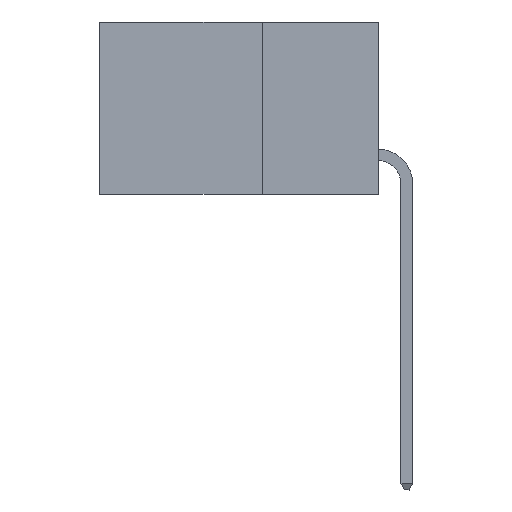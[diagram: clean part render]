
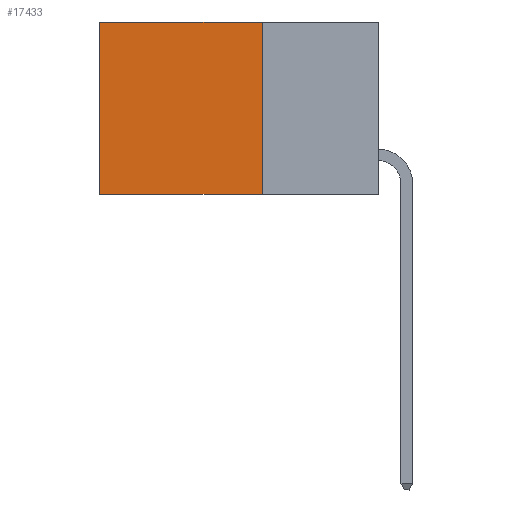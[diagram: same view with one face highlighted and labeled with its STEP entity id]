
A CAD part, left-side view. The second image highlights one B-rep face of the part: STEP entity #17433.
In plain terms, the highlighted planar face has unit normal (-1, 0, 0).
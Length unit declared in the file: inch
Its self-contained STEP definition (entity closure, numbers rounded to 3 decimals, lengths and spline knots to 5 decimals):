
#5151 = VECTOR ( 'NONE', #5388, 39.37008 ) ;
#5304 = CARTESIAN_POINT ( 'NONE',  ( 0.298, 0.25, 0. ) ) ;
#5388 = DIRECTION ( 'NONE',  ( 0., 1., 0. ) ) ;
#5449 = VECTOR ( 'NONE', #15391, 39.37008 ) ;
#6248 = CARTESIAN_POINT ( 'NONE',  ( 0.298, 0.6, 0. ) ) ;
#6338 = VERTEX_POINT ( 'NONE', #20935 ) ;
#7068 = ORIENTED_EDGE ( 'NONE', *, *, #19217, .F. ) ;
#7825 = ORIENTED_EDGE ( 'NONE', *, *, #17321, .T. ) ;
#8669 = EDGE_CURVE ( 'NONE', #17113, #14033, #10089, .T. ) ;
#9116 = VECTOR ( 'NONE', #25339, 39.37008 ) ;
#9495 = ORIENTED_EDGE ( 'NONE', *, *, #8669, .T. ) ;
#9577 = CARTESIAN_POINT ( 'NONE',  ( 0.298, 0.25, 0. ) ) ;
#10061 = EDGE_CURVE ( 'NONE', #6338, #14033, #15843, .T. ) ;
#10089 = LINE ( 'NONE', #6248, #9116 ) ;
#11891 = CARTESIAN_POINT ( 'NONE',  ( 0.298, 0.25, 0. ) ) ;
#12530 = CARTESIAN_POINT ( 'NONE',  ( 0.298, 0.6, 0. ) ) ;
#12676 = ORIENTED_EDGE ( 'NONE', *, *, #10061, .F. ) ;
#13396 = EDGE_LOOP ( 'NONE', ( #9495, #12676, #7068, #7825 ) ) ;
#13481 = CARTESIAN_POINT ( 'NONE',  ( 0.298, 0.25, -0.37 ) ) ;
#14033 = VERTEX_POINT ( 'NONE', #27015 ) ;
#15391 = DIRECTION ( 'NONE',  ( 0., 1., 0. ) ) ;
#15843 = LINE ( 'NONE', #13481, #5449 ) ;
#17113 = VERTEX_POINT ( 'NONE', #12530 ) ;
#17321 = EDGE_CURVE ( 'NONE', #18151, #17113, #27006, .T. ) ;
#17433 = ADVANCED_FACE ( 'NONE', ( #26339 ), #23922, .F. ) ;
#18151 = VERTEX_POINT ( 'NONE', #18323 ) ;
#18323 = CARTESIAN_POINT ( 'NONE',  ( 0.298, 0.25, 0. ) ) ;
#19217 = EDGE_CURVE ( 'NONE', #18151, #6338, #20966, .T. ) ;
#19815 = DIRECTION ( 'NONE',  ( 1., 0., 0. ) ) ;
#20935 = CARTESIAN_POINT ( 'NONE',  ( 0.298, 0.25, -0.37 ) ) ;
#20966 = LINE ( 'NONE', #11891, #26202 ) ;
#21256 = AXIS2_PLACEMENT_3D ( 'NONE', #5304, #19815, #24859 ) ;
#22048 = DIRECTION ( 'NONE',  ( 0., 0., -1. ) ) ;
#23922 = PLANE ( 'NONE',  #21256 ) ;
#24859 = DIRECTION ( 'NONE',  ( 0., 0., -1. ) ) ;
#25339 = DIRECTION ( 'NONE',  ( 0., 0., -1. ) ) ;
#26202 = VECTOR ( 'NONE', #22048, 39.37008 ) ;
#26339 = FACE_OUTER_BOUND ( 'NONE', #13396, .T. ) ;
#27006 = LINE ( 'NONE', #9577, #5151 ) ;
#27015 = CARTESIAN_POINT ( 'NONE',  ( 0.298, 0.6, -0.37 ) ) ;
